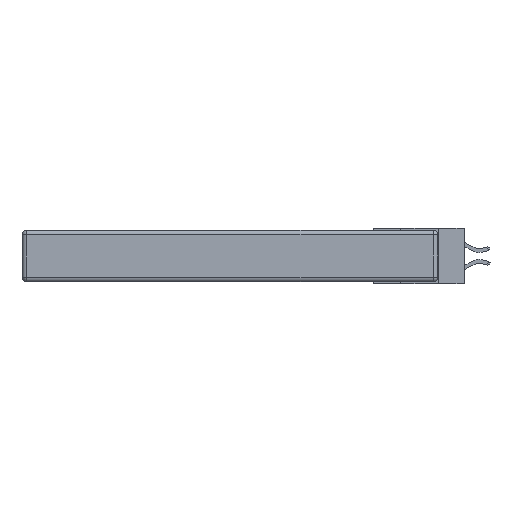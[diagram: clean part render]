
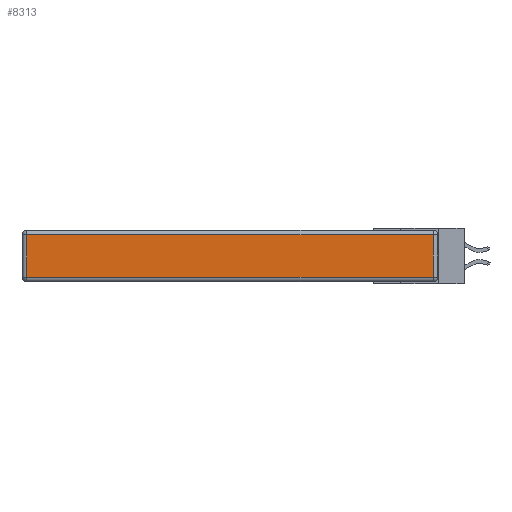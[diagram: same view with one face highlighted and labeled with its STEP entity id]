
A CAD part, left-side view. The second image highlights one B-rep face of the part: STEP entity #8313.
In plain terms, the highlighted planar face has unit normal (-1, 0, 0).
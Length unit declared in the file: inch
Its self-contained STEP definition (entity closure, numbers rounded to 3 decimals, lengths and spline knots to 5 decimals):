
#142 = ORIENTED_EDGE ( 'NONE', *, *, #17192, .T. ) ;
#206 = LINE ( 'NONE', #15441, #1358 ) ;
#284 = VECTOR ( 'NONE', #11218, 39.37008 ) ;
#511 = AXIS2_PLACEMENT_3D ( 'NONE', #1065, #18979, #4114 ) ;
#610 = CARTESIAN_POINT ( 'NONE',  ( 0., 2.75, -0.03 ) ) ;
#1009 = CARTESIAN_POINT ( 'NONE',  ( 0., 0.03, -0.313 ) ) ;
#1065 = CARTESIAN_POINT ( 'NONE',  ( 0., 0., -0.343 ) ) ;
#1358 = VECTOR ( 'NONE', #6386, 39.37008 ) ;
#2136 = ORIENTED_EDGE ( 'NONE', *, *, #8485, .T. ) ;
#3269 = DIRECTION ( 'NONE',  ( 0., -1., 0. ) ) ;
#4114 = DIRECTION ( 'NONE',  ( 0., 0., 1. ) ) ;
#4481 = VECTOR ( 'NONE', #3269, 39.37008 ) ;
#4597 = CARTESIAN_POINT ( 'NONE',  ( 0., 2.72, -0.313 ) ) ;
#4670 = EDGE_LOOP ( 'NONE', ( #142, #10756, #16723, #2136 ) ) ;
#4957 = CARTESIAN_POINT ( 'NONE',  ( 0., 2.72, -0.03 ) ) ;
#5428 = PLANE ( 'NONE',  #511 ) ;
#6386 = DIRECTION ( 'NONE',  ( 0., 0., 1. ) ) ;
#6754 = VERTEX_POINT ( 'NONE', #4957 ) ;
#8009 = FACE_OUTER_BOUND ( 'NONE', #4670, .T. ) ;
#8145 = EDGE_CURVE ( 'NONE', #11586, #8688, #206, .T. ) ;
#8313 = ADVANCED_FACE ( 'NONE', ( #8009 ), #5428, .T. ) ;
#8332 = LINE ( 'NONE', #610, #284 ) ;
#8485 = EDGE_CURVE ( 'NONE', #6754, #9035, #15551, .T. ) ;
#8534 = LINE ( 'NONE', #18341, #4481 ) ;
#8688 = VERTEX_POINT ( 'NONE', #18937 ) ;
#9035 = VERTEX_POINT ( 'NONE', #4597 ) ;
#10756 = ORIENTED_EDGE ( 'NONE', *, *, #8145, .T. ) ;
#11218 = DIRECTION ( 'NONE',  ( 0., 1., 0. ) ) ;
#11586 = VERTEX_POINT ( 'NONE', #1009 ) ;
#13577 = CARTESIAN_POINT ( 'NONE',  ( 0., 2.72, -0.343 ) ) ;
#13770 = DIRECTION ( 'NONE',  ( 0., 0., -1. ) ) ;
#15083 = VECTOR ( 'NONE', #13770, 39.37008 ) ;
#15441 = CARTESIAN_POINT ( 'NONE',  ( 0., 0.03, -0.343 ) ) ;
#15551 = LINE ( 'NONE', #13577, #15083 ) ;
#16480 = EDGE_CURVE ( 'NONE', #8688, #6754, #8332, .T. ) ;
#16723 = ORIENTED_EDGE ( 'NONE', *, *, #16480, .T. ) ;
#17192 = EDGE_CURVE ( 'NONE', #9035, #11586, #8534, .T. ) ;
#18341 = CARTESIAN_POINT ( 'NONE',  ( 0., 0., -0.313 ) ) ;
#18937 = CARTESIAN_POINT ( 'NONE',  ( 0., 0.03, -0.03 ) ) ;
#18979 = DIRECTION ( 'NONE',  ( -1., 0., 0. ) ) ;
